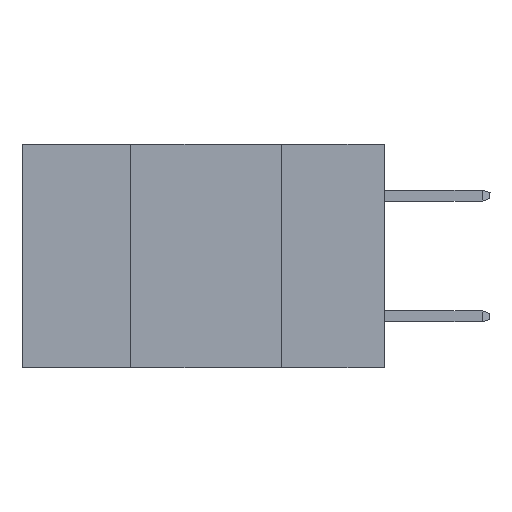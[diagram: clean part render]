
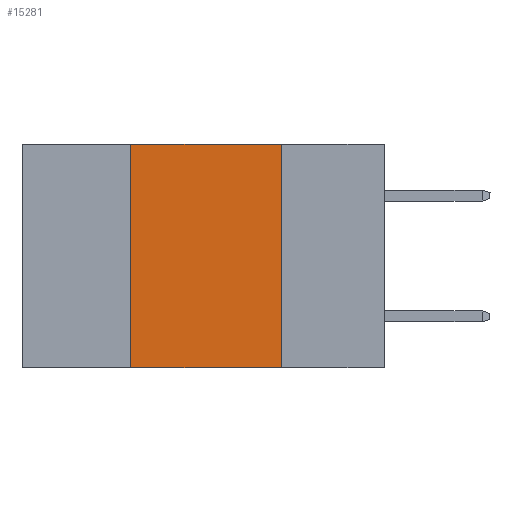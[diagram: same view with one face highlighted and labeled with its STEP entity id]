
A CAD part, left-side view. The second image highlights one B-rep face of the part: STEP entity #15281.
In plain terms, the highlighted planar face has unit normal (-1, 0, 0).
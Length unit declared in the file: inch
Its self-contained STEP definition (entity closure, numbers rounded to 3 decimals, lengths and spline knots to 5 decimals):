
#456 = VERTEX_POINT ( 'NONE', #17045 ) ;
#1647 = EDGE_CURVE ( 'NONE', #10282, #10057, #26198, .T. ) ;
#2917 = AXIS2_PLACEMENT_3D ( 'NONE', #23473, #28496, #13351 ) ;
#3201 = FACE_OUTER_BOUND ( 'NONE', #12634, .T. ) ;
#3394 = EDGE_CURVE ( 'NONE', #24963, #456, #13556, .T. ) ;
#5934 = CARTESIAN_POINT ( 'NONE',  ( 0., 0.42, -0.37 ) ) ;
#6449 = LINE ( 'NONE', #22788, #25961 ) ;
#6956 = VECTOR ( 'NONE', #7270, 39.37008 ) ;
#7270 = DIRECTION ( 'NONE',  ( 0., -1., 0. ) ) ;
#8506 = EDGE_CURVE ( 'NONE', #10282, #456, #6449, .T. ) ;
#10057 = VERTEX_POINT ( 'NONE', #12645 ) ;
#10282 = VERTEX_POINT ( 'NONE', #5934 ) ;
#10777 = PLANE ( 'NONE',  #2917 ) ;
#11869 = CARTESIAN_POINT ( 'NONE',  ( 0., 0.17, 0. ) ) ;
#12634 = EDGE_LOOP ( 'NONE', ( #24970, #25751, #26511, #19805 ) ) ;
#12645 = CARTESIAN_POINT ( 'NONE',  ( 0., 0.42, 0. ) ) ;
#13351 = DIRECTION ( 'NONE',  ( 0., 0., -1. ) ) ;
#13487 = VECTOR ( 'NONE', #18372, 39.37008 ) ;
#13556 = LINE ( 'NONE', #15002, #20692 ) ;
#14079 = DIRECTION ( 'NONE',  ( 0., 0., -1. ) ) ;
#15002 = CARTESIAN_POINT ( 'NONE',  ( 0., 0.17, 0. ) ) ;
#15281 = ADVANCED_FACE ( 'NONE', ( #3201 ), #10777, .F. ) ;
#17045 = CARTESIAN_POINT ( 'NONE',  ( 0., 0.17, -0.37 ) ) ;
#18229 = CARTESIAN_POINT ( 'NONE',  ( 0., 0.42, 0. ) ) ;
#18372 = DIRECTION ( 'NONE',  ( 0., 0., 1. ) ) ;
#19805 = ORIENTED_EDGE ( 'NONE', *, *, #8506, .T. ) ;
#20681 = EDGE_CURVE ( 'NONE', #10057, #24963, #27235, .T. ) ;
#20692 = VECTOR ( 'NONE', #14079, 39.37008 ) ;
#22788 = CARTESIAN_POINT ( 'NONE',  ( 0., 0.6, -0.37 ) ) ;
#23473 = CARTESIAN_POINT ( 'NONE',  ( 0., 0.6, 0. ) ) ;
#24963 = VERTEX_POINT ( 'NONE', #11869 ) ;
#24970 = ORIENTED_EDGE ( 'NONE', *, *, #3394, .F. ) ;
#25751 = ORIENTED_EDGE ( 'NONE', *, *, #20681, .F. ) ;
#25961 = VECTOR ( 'NONE', #32677, 39.37008 ) ;
#26198 = LINE ( 'NONE', #18229, #13487 ) ;
#26511 = ORIENTED_EDGE ( 'NONE', *, *, #1647, .F. ) ;
#27235 = LINE ( 'NONE', #27574, #6956 ) ;
#27574 = CARTESIAN_POINT ( 'NONE',  ( 0., 0.6, 0. ) ) ;
#28496 = DIRECTION ( 'NONE',  ( 1., 0., 0. ) ) ;
#32677 = DIRECTION ( 'NONE',  ( 0., -1., 0. ) ) ;
